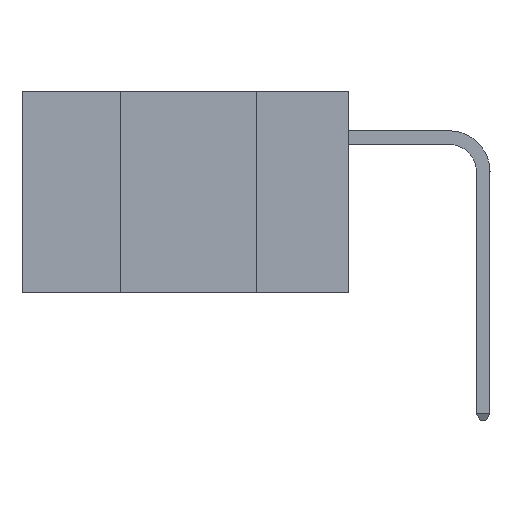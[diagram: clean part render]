
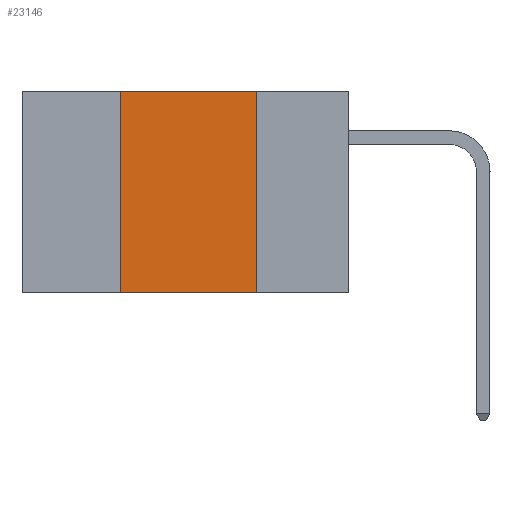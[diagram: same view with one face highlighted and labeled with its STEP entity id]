
A CAD part, left-side view. The second image highlights one B-rep face of the part: STEP entity #23146.
In plain terms, the highlighted planar face has unit normal (-1, 0, 0).
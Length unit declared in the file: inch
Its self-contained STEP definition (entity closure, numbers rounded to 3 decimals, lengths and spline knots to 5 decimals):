
#759 = EDGE_CURVE ( 'NONE', #10061, #29425, #20868, .T. ) ;
#1664 = DIRECTION ( 'NONE',  ( 0., -1., 0. ) ) ;
#3579 = CARTESIAN_POINT ( 'NONE',  ( 0., 0.17, 0. ) ) ;
#4191 = VECTOR ( 'NONE', #13749, 39.37008 ) ;
#4406 = VECTOR ( 'NONE', #1664, 39.37008 ) ;
#4658 = VECTOR ( 'NONE', #27640, 39.37008 ) ;
#5160 = LINE ( 'NONE', #13864, #4406 ) ;
#6231 = ORIENTED_EDGE ( 'NONE', *, *, #759, .F. ) ;
#7023 = VERTEX_POINT ( 'NONE', #22857 ) ;
#7159 = CARTESIAN_POINT ( 'NONE',  ( 0., 0.6, 0. ) ) ;
#9613 = DIRECTION ( 'NONE',  ( 1., 0., 0. ) ) ;
#10060 = FACE_OUTER_BOUND ( 'NONE', #31088, .T. ) ;
#10061 = VERTEX_POINT ( 'NONE', #25678 ) ;
#10263 = CARTESIAN_POINT ( 'NONE',  ( 0., 0.42, 0. ) ) ;
#11170 = LINE ( 'NONE', #3579, #4658 ) ;
#11298 = CARTESIAN_POINT ( 'NONE',  ( 0., 0.6, 0. ) ) ;
#13749 = DIRECTION ( 'NONE',  ( 0., -1., 0. ) ) ;
#13864 = CARTESIAN_POINT ( 'NONE',  ( 0., 0.6, -0.37 ) ) ;
#14408 = PLANE ( 'NONE',  #25877 ) ;
#14515 = VECTOR ( 'NONE', #27192, 39.37008 ) ;
#17658 = ORIENTED_EDGE ( 'NONE', *, *, #28723, .F. ) ;
#20635 = ORIENTED_EDGE ( 'NONE', *, *, #31015, .T. ) ;
#20868 = LINE ( 'NONE', #10263, #14515 ) ;
#22857 = CARTESIAN_POINT ( 'NONE',  ( 0., 0.17, -0.37 ) ) ;
#23146 = ADVANCED_FACE ( 'NONE', ( #10060 ), #14408, .F. ) ;
#23228 = ORIENTED_EDGE ( 'NONE', *, *, #23490, .F. ) ;
#23490 = EDGE_CURVE ( 'NONE', #27522, #7023, #11170, .T. ) ;
#25678 = CARTESIAN_POINT ( 'NONE',  ( 0., 0.42, -0.37 ) ) ;
#25731 = LINE ( 'NONE', #11298, #4191 ) ;
#25877 = AXIS2_PLACEMENT_3D ( 'NONE', #7159, #9613, #26361 ) ;
#25934 = CARTESIAN_POINT ( 'NONE',  ( 0., 0.17, 0. ) ) ;
#26361 = DIRECTION ( 'NONE',  ( 0., 0., -1. ) ) ;
#27192 = DIRECTION ( 'NONE',  ( 0., 0., 1. ) ) ;
#27522 = VERTEX_POINT ( 'NONE', #25934 ) ;
#27640 = DIRECTION ( 'NONE',  ( 0., 0., -1. ) ) ;
#28723 = EDGE_CURVE ( 'NONE', #29425, #27522, #25731, .T. ) ;
#29425 = VERTEX_POINT ( 'NONE', #30532 ) ;
#30532 = CARTESIAN_POINT ( 'NONE',  ( 0., 0.42, 0. ) ) ;
#31015 = EDGE_CURVE ( 'NONE', #10061, #7023, #5160, .T. ) ;
#31088 = EDGE_LOOP ( 'NONE', ( #23228, #17658, #6231, #20635 ) ) ;
